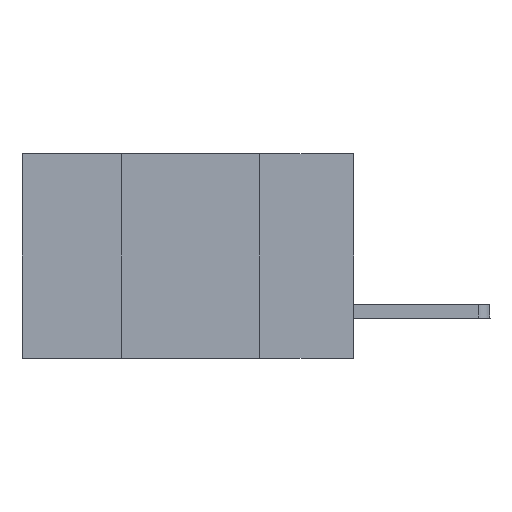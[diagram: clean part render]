
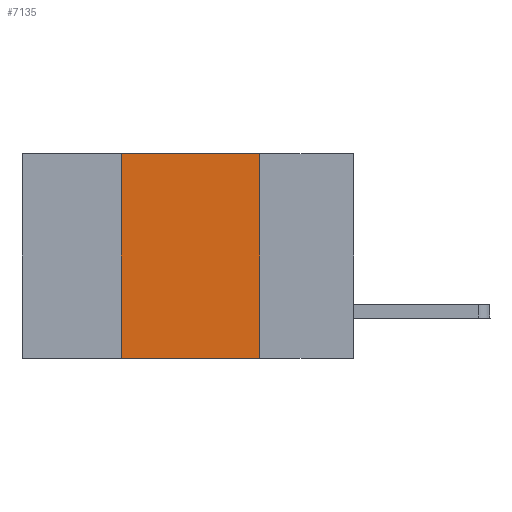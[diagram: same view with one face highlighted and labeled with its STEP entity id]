
A CAD part, left-side view. The second image highlights one B-rep face of the part: STEP entity #7135.
In plain terms, the highlighted planar face has unit normal (-1, 0, 0).
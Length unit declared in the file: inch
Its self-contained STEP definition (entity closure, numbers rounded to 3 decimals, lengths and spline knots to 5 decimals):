
#1 = EDGE_CURVE ( 'NONE', #5720, #6713, #3927, .T. ) ;
#544 = VECTOR ( 'NONE', #9800, 39.37008 ) ;
#763 = AXIS2_PLACEMENT_3D ( 'NONE', #5085, #12257, #13453 ) ;
#1417 = LINE ( 'NONE', #6961, #10413 ) ;
#1674 = EDGE_CURVE ( 'NONE', #4052, #12843, #2898, .T. ) ;
#2096 = CARTESIAN_POINT ( 'NONE',  ( 0., 0.17, 0. ) ) ;
#2721 = VECTOR ( 'NONE', #12352, 39.37008 ) ;
#2898 = LINE ( 'NONE', #5020, #2721 ) ;
#3610 = EDGE_LOOP ( 'NONE', ( #12444, #14399, #14050, #6227 ) ) ;
#3861 = PLANE ( 'NONE',  #763 ) ;
#3927 = LINE ( 'NONE', #8591, #544 ) ;
#4052 = VERTEX_POINT ( 'NONE', #12621 ) ;
#5020 = CARTESIAN_POINT ( 'NONE',  ( 0., 0.6, -0.37 ) ) ;
#5085 = CARTESIAN_POINT ( 'NONE',  ( 0., 0.6, 0. ) ) ;
#5720 = VERTEX_POINT ( 'NONE', #9037 ) ;
#6224 = FACE_OUTER_BOUND ( 'NONE', #3610, .T. ) ;
#6227 = ORIENTED_EDGE ( 'NONE', *, *, #1674, .T. ) ;
#6485 = CARTESIAN_POINT ( 'NONE',  ( 0., 0.17, 0. ) ) ;
#6559 = LINE ( 'NONE', #6485, #10098 ) ;
#6713 = VERTEX_POINT ( 'NONE', #2096 ) ;
#6961 = CARTESIAN_POINT ( 'NONE',  ( 0., 0.42, 0. ) ) ;
#7135 = ADVANCED_FACE ( 'NONE', ( #6224 ), #3861, .F. ) ;
#7178 = CARTESIAN_POINT ( 'NONE',  ( 0., 0.17, -0.37 ) ) ;
#8591 = CARTESIAN_POINT ( 'NONE',  ( 0., 0.6, 0. ) ) ;
#9037 = CARTESIAN_POINT ( 'NONE',  ( 0., 0.42, 0. ) ) ;
#9359 = DIRECTION ( 'NONE',  ( 0., 0., 1. ) ) ;
#9415 = EDGE_CURVE ( 'NONE', #6713, #12843, #6559, .T. ) ;
#9800 = DIRECTION ( 'NONE',  ( 0., -1., 0. ) ) ;
#10092 = DIRECTION ( 'NONE',  ( 0., 0., -1. ) ) ;
#10098 = VECTOR ( 'NONE', #10092, 39.37008 ) ;
#10413 = VECTOR ( 'NONE', #9359, 39.37008 ) ;
#11233 = EDGE_CURVE ( 'NONE', #4052, #5720, #1417, .T. ) ;
#12257 = DIRECTION ( 'NONE',  ( 1., 0., 0. ) ) ;
#12352 = DIRECTION ( 'NONE',  ( 0., -1., 0. ) ) ;
#12444 = ORIENTED_EDGE ( 'NONE', *, *, #9415, .F. ) ;
#12621 = CARTESIAN_POINT ( 'NONE',  ( 0., 0.42, -0.37 ) ) ;
#12843 = VERTEX_POINT ( 'NONE', #7178 ) ;
#13453 = DIRECTION ( 'NONE',  ( 0., 0., -1. ) ) ;
#14050 = ORIENTED_EDGE ( 'NONE', *, *, #11233, .F. ) ;
#14399 = ORIENTED_EDGE ( 'NONE', *, *, #1, .F. ) ;
